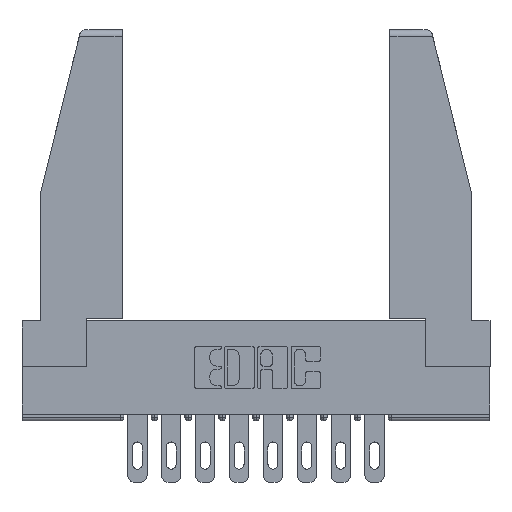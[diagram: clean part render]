
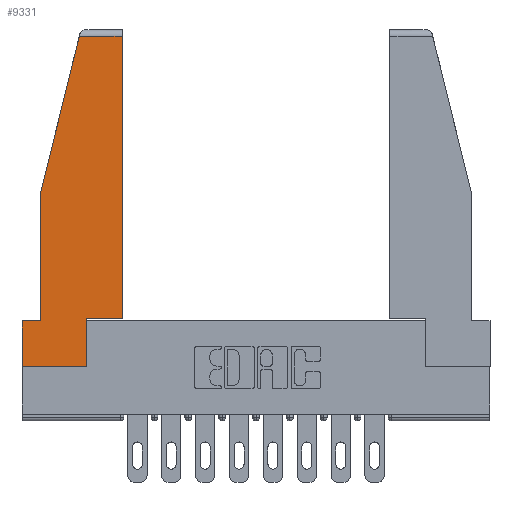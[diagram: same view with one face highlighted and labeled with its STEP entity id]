
A CAD part, top view. The second image highlights one B-rep face of the part: STEP entity #9331.
In plain terms, the highlighted planar face has unit normal (0, 0, 1).
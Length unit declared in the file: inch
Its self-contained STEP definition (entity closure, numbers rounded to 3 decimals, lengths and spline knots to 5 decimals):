
#59 = CARTESIAN_POINT ( 'NONE',  ( 0., 0.21, 0. ) ) ;
#556 = VERTEX_POINT ( 'NONE', #1148 ) ;
#590 = VECTOR ( 'NONE', #7575, 39.37008 ) ;
#593 = EDGE_CURVE ( 'NONE', #3151, #10926, #11647, .T. ) ;
#1148 = CARTESIAN_POINT ( 'NONE',  ( 0., 0.21, 0. ) ) ;
#1478 = CARTESIAN_POINT ( 'NONE',  ( 0.2636, 1.52, 0. ) ) ;
#1586 = EDGE_CURVE ( 'NONE', #3057, #14393, #7401, .T. ) ;
#1783 = EDGE_CURVE ( 'NONE', #8891, #3057, #2933, .T. ) ;
#1871 = CARTESIAN_POINT ( 'NONE',  ( 0.297, 0.223, 0. ) ) ;
#1939 = PLANE ( 'NONE',  #11795 ) ;
#2102 = CARTESIAN_POINT ( 'NONE',  ( 0.461, 1.52, 0. ) ) ;
#2289 = ORIENTED_EDGE ( 'NONE', *, *, #14659, .T. ) ;
#2688 = ORIENTED_EDGE ( 'NONE', *, *, #2782, .T. ) ;
#2782 = EDGE_CURVE ( 'NONE', #556, #3151, #5827, .T. ) ;
#2933 = LINE ( 'NONE', #14063, #11987 ) ;
#3057 = VERTEX_POINT ( 'NONE', #7176 ) ;
#3146 = VECTOR ( 'NONE', #11645, 39.37008 ) ;
#3151 = VERTEX_POINT ( 'NONE', #10412 ) ;
#3260 = ORIENTED_EDGE ( 'NONE', *, *, #15033, .T. ) ;
#3382 = ORIENTED_EDGE ( 'NONE', *, *, #13256, .T. ) ;
#3390 = LINE ( 'NONE', #5702, #10463 ) ;
#3428 = VECTOR ( 'NONE', #11719, 39.37008 ) ;
#3809 = CARTESIAN_POINT ( 'NONE',  ( 0.461, 0.223, 0. ) ) ;
#3847 = VECTOR ( 'NONE', #6141, 39.37008 ) ;
#3980 = CARTESIAN_POINT ( 'NONE',  ( 0.461, 0.223, 0. ) ) ;
#4184 = LINE ( 'NONE', #9503, #10148 ) ;
#4620 = DIRECTION ( 'NONE',  ( -1., 0., 0. ) ) ;
#5052 = ORIENTED_EDGE ( 'NONE', *, *, #593, .T. ) ;
#5702 = CARTESIAN_POINT ( 'NONE',  ( 0.297, 0., 0. ) ) ;
#5827 = LINE ( 'NONE', #59, #14903 ) ;
#6141 = DIRECTION ( 'NONE',  ( 0., -1., 0. ) ) ;
#7043 = CARTESIAN_POINT ( 'NONE',  ( 0.297, 0.223, 0. ) ) ;
#7083 = DIRECTION ( 'NONE',  ( 0., 1., 0. ) ) ;
#7176 = CARTESIAN_POINT ( 'NONE',  ( 0.086, 0.8, 0. ) ) ;
#7401 = LINE ( 'NONE', #13201, #3847 ) ;
#7575 = DIRECTION ( 'NONE',  ( 0., 1., 0. ) ) ;
#7739 = ORIENTED_EDGE ( 'NONE', *, *, #1783, .T. ) ;
#8891 = VERTEX_POINT ( 'NONE', #1478 ) ;
#9331 = ADVANCED_FACE ( 'NONE', ( #10699 ), #1939, .T. ) ;
#9416 = DIRECTION ( 'NONE',  ( -0.239, -0.971, 0. ) ) ;
#9503 = CARTESIAN_POINT ( 'NONE',  ( 0., 0.21, 0. ) ) ;
#9831 = DIRECTION ( 'NONE',  ( 0., -1., 0. ) ) ;
#10148 = VECTOR ( 'NONE', #11850, 39.37008 ) ;
#10326 = EDGE_CURVE ( 'NONE', #10926, #14943, #3390, .T. ) ;
#10383 = DIRECTION ( 'NONE',  ( 1., 0., 0. ) ) ;
#10412 = CARTESIAN_POINT ( 'NONE',  ( 0., 0., 0. ) ) ;
#10463 = VECTOR ( 'NONE', #7083, 39.37008 ) ;
#10490 = CARTESIAN_POINT ( 'NONE',  ( 0., 0., 0. ) ) ;
#10493 = ORIENTED_EDGE ( 'NONE', *, *, #10326, .T. ) ;
#10699 = FACE_OUTER_BOUND ( 'NONE', #14521, .T. ) ;
#10871 = VERTEX_POINT ( 'NONE', #3809 ) ;
#10926 = VERTEX_POINT ( 'NONE', #15136 ) ;
#11181 = CARTESIAN_POINT ( 'NONE',  ( 0.086, 0.21, 0. ) ) ;
#11315 = VECTOR ( 'NONE', #4620, 39.37008 ) ;
#11533 = CARTESIAN_POINT ( 'NONE',  ( 0., 0., 0. ) ) ;
#11645 = DIRECTION ( 'NONE',  ( 1., 0., 0. ) ) ;
#11647 = LINE ( 'NONE', #10490, #3146 ) ;
#11719 = DIRECTION ( 'NONE',  ( 1., 0., 0. ) ) ;
#11795 = AXIS2_PLACEMENT_3D ( 'NONE', #11533, #13851, #10383 ) ;
#11850 = DIRECTION ( 'NONE',  ( -1., 0., 0. ) ) ;
#11886 = EDGE_CURVE ( 'NONE', #14099, #8891, #14834, .T. ) ;
#11987 = VECTOR ( 'NONE', #9416, 39.37008 ) ;
#12221 = ORIENTED_EDGE ( 'NONE', *, *, #11886, .T. ) ;
#13201 = CARTESIAN_POINT ( 'NONE',  ( 0.086, 0.8, 0. ) ) ;
#13256 = EDGE_CURVE ( 'NONE', #10871, #14099, #14033, .T. ) ;
#13851 = DIRECTION ( 'NONE',  ( 0., 0., 1. ) ) ;
#14033 = LINE ( 'NONE', #3980, #590 ) ;
#14063 = CARTESIAN_POINT ( 'NONE',  ( 0.271, 1.55, 0. ) ) ;
#14099 = VERTEX_POINT ( 'NONE', #2102 ) ;
#14190 = ORIENTED_EDGE ( 'NONE', *, *, #1586, .T. ) ;
#14393 = VERTEX_POINT ( 'NONE', #11181 ) ;
#14521 = EDGE_LOOP ( 'NONE', ( #3382, #12221, #7739, #14190, #2289, #2688, #5052, #10493, #3260 ) ) ;
#14659 = EDGE_CURVE ( 'NONE', #14393, #556, #4184, .T. ) ;
#14823 = CARTESIAN_POINT ( 'NONE',  ( 0., 1.52, 0. ) ) ;
#14834 = LINE ( 'NONE', #14823, #11315 ) ;
#14903 = VECTOR ( 'NONE', #9831, 39.37008 ) ;
#14907 = LINE ( 'NONE', #7043, #3428 ) ;
#14943 = VERTEX_POINT ( 'NONE', #1871 ) ;
#15033 = EDGE_CURVE ( 'NONE', #14943, #10871, #14907, .T. ) ;
#15136 = CARTESIAN_POINT ( 'NONE',  ( 0.297, 0., 0. ) ) ;
